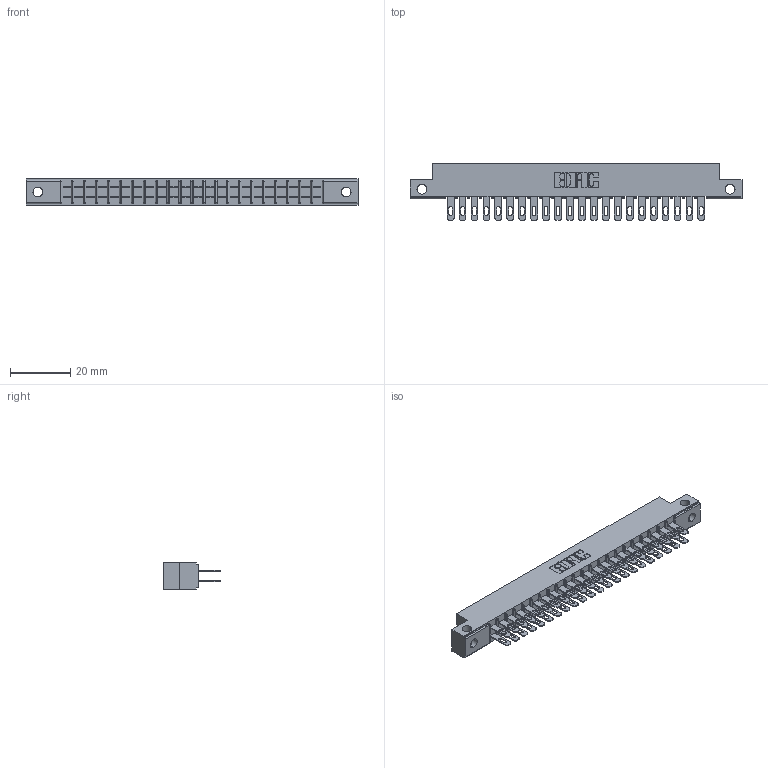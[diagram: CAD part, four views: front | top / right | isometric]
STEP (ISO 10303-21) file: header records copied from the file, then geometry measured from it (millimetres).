
FILE_DESCRIPTION (( 'STEP AP203' ), '1' );
FILE_NAME ('305-044-500-512.STEP', '2020-09-19T22:14:37', ( '' ), ( '' ), 'SwSTEP 2.0', 'SolidWorks 2020', '' );
FILE_SCHEMA (( 'CONFIG_CONTROL_DESIGN' ));
Length unit declared in the file: inch
Products named in the file (3): 305 Part_.128 Dia; 305-044-500-512; 305-290-001_500
Assembly tree (45 placements, depth 2):
  305-044-500-512
    305 Part_.128 Dia
    305-290-001_500  x44
Bounding box: 110.19 x 18.85 x 8.71 mm (x, y, z)
Volume: 6603.2 mm3; surface area: 13926.9 mm2
Topology: 45 solids, 45 shells, 2328 faces, 6666 edges, 4320 vertices
Faces by surface type: plane 1300, cylinder 940, sphere 88
Entity records: 26683 total; most frequent: CARTESIAN_POINT 4464, ORIENTED_EDGE 4384, DIRECTION 4276, EDGE_CURVE 2192, VECTOR 1732, LINE 1732, VERTEX_POINT 1396, AXIS2_PLACEMENT_3D 1272
